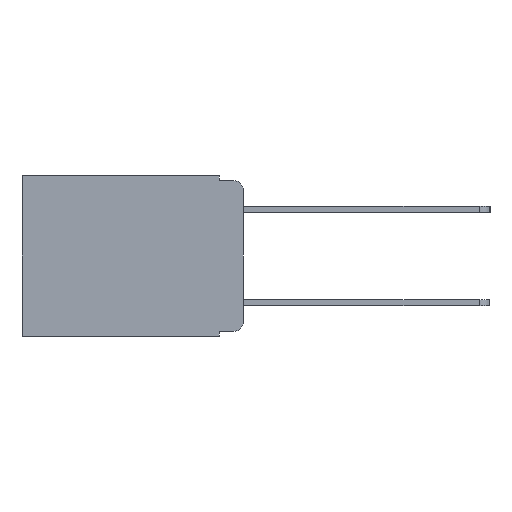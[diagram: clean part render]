
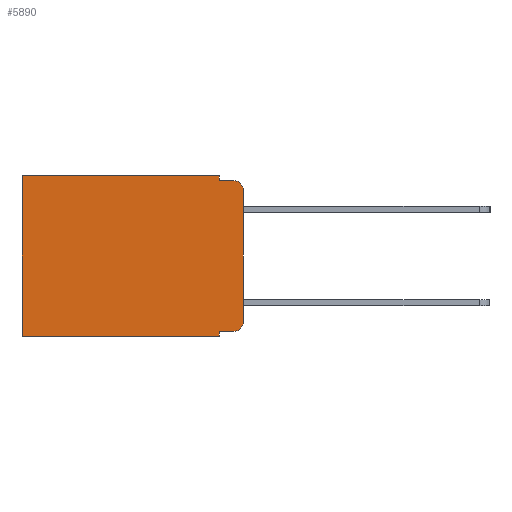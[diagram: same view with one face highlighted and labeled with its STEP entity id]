
A CAD part, left-side view. The second image highlights one B-rep face of the part: STEP entity #5890.
In plain terms, the highlighted planar face has unit normal (-1, 0, 0).
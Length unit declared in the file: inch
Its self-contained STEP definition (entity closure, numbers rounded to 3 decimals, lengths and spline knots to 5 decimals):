
#100 = CARTESIAN_POINT ( 'NONE',  ( 0.298, 0., 0. ) ) ;
#235 = VERTEX_POINT ( 'NONE', #10505 ) ;
#363 = ORIENTED_EDGE ( 'NONE', *, *, #10408, .T. ) ;
#366 = EDGE_CURVE ( 'NONE', #2660, #1047, #8768, .T. ) ;
#435 = EDGE_CURVE ( 'NONE', #1934, #4806, #10610, .T. ) ;
#436 = ORIENTED_EDGE ( 'NONE', *, *, #435, .T. ) ;
#589 = VECTOR ( 'NONE', #9403, 39.37008 ) ;
#624 = ORIENTED_EDGE ( 'NONE', *, *, #366, .F. ) ;
#660 = VERTEX_POINT ( 'NONE', #872 ) ;
#872 = CARTESIAN_POINT ( 'NONE',  ( 0.298, 0.051, -0.333 ) ) ;
#1047 = VERTEX_POINT ( 'NONE', #6591 ) ;
#1181 = DIRECTION ( 'NONE',  ( 0., 0., -1. ) ) ;
#1184 = CARTESIAN_POINT ( 'NONE',  ( 0.298, 0.051, 0. ) ) ;
#1811 = DIRECTION ( 'NONE',  ( 0., 1., 0. ) ) ;
#1934 = VERTEX_POINT ( 'NONE', #4627 ) ;
#2056 = VECTOR ( 'NONE', #4995, 39.37008 ) ;
#2133 = AXIS2_PLACEMENT_3D ( 'NONE', #8592, #3568, #9383 ) ;
#2230 = DIRECTION ( 'NONE',  ( 0., 0., -1. ) ) ;
#2364 = VERTEX_POINT ( 'NONE', #4987 ) ;
#2460 = AXIS2_PLACEMENT_3D ( 'NONE', #4504, #6035, #4057 ) ;
#2660 = VERTEX_POINT ( 'NONE', #5767 ) ;
#2763 = LINE ( 'NONE', #4323, #9146 ) ;
#2935 = LINE ( 'NONE', #100, #589 ) ;
#3089 = AXIS2_PLACEMENT_3D ( 'NONE', #3874, #6316, #7940 ) ;
#3096 = CARTESIAN_POINT ( 'NONE',  ( 0.298, 0.051, 0. ) ) ;
#3352 = CIRCLE ( 'NONE', #2133, 0.02 ) ;
#3515 = ORIENTED_EDGE ( 'NONE', *, *, #6199, .F. ) ;
#3568 = DIRECTION ( 'NONE',  ( -1., 0., 0. ) ) ;
#3852 = LINE ( 'NONE', #9839, #8577 ) ;
#3874 = CARTESIAN_POINT ( 'NONE',  ( 0.298, 0.02, -0.313 ) ) ;
#4001 = LINE ( 'NONE', #10686, #8207 ) ;
#4057 = DIRECTION ( 'NONE',  ( 0., 0., -1. ) ) ;
#4323 = CARTESIAN_POINT ( 'NONE',  ( 0.298, 0., 0. ) ) ;
#4504 = CARTESIAN_POINT ( 'NONE',  ( 0.298, 0., 0. ) ) ;
#4610 = CARTESIAN_POINT ( 'NONE',  ( 0.298, 0., -0.03 ) ) ;
#4627 = CARTESIAN_POINT ( 'NONE',  ( 0.298, 0.02, -0.333 ) ) ;
#4632 = VECTOR ( 'NONE', #2230, 39.37008 ) ;
#4806 = VERTEX_POINT ( 'NONE', #10694 ) ;
#4987 = CARTESIAN_POINT ( 'NONE',  ( 0.298, 0.051, 0. ) ) ;
#4995 = DIRECTION ( 'NONE',  ( 0., 1., 0. ) ) ;
#5471 = LINE ( 'NONE', #1184, #6018 ) ;
#5699 = VERTEX_POINT ( 'NONE', #10056 ) ;
#5726 = DIRECTION ( 'NONE',  ( 0., -1., 0. ) ) ;
#5732 = CARTESIAN_POINT ( 'NONE',  ( 0.298, 0., -0.343 ) ) ;
#5767 = CARTESIAN_POINT ( 'NONE',  ( 0.298, 0.051, -0.343 ) ) ;
#5837 = DIRECTION ( 'NONE',  ( 0., 0., -1. ) ) ;
#5890 = ADVANCED_FACE ( 'NONE', ( #9363 ), #7593, .F. ) ;
#5957 = EDGE_CURVE ( 'NONE', #9773, #235, #10722, .T. ) ;
#6018 = VECTOR ( 'NONE', #1181, 39.37008 ) ;
#6035 = DIRECTION ( 'NONE',  ( 1., 0., 0. ) ) ;
#6199 = EDGE_CURVE ( 'NONE', #2364, #9773, #5471, .T. ) ;
#6316 = DIRECTION ( 'NONE',  ( -1., 0., 0. ) ) ;
#6423 = ORIENTED_EDGE ( 'NONE', *, *, #5957, .F. ) ;
#6591 = CARTESIAN_POINT ( 'NONE',  ( 0.298, 0.473, -0.343 ) ) ;
#6660 = ORIENTED_EDGE ( 'NONE', *, *, #8066, .T. ) ;
#6733 = EDGE_LOOP ( 'NONE', ( #8802, #6660, #6423, #3515, #7667, #363, #624, #8379, #7377, #436 ) ) ;
#7128 = VERTEX_POINT ( 'NONE', #4610 ) ;
#7339 = DIRECTION ( 'NONE',  ( 0., -1., 0. ) ) ;
#7377 = ORIENTED_EDGE ( 'NONE', *, *, #8397, .T. ) ;
#7593 = PLANE ( 'NONE',  #2460 ) ;
#7667 = ORIENTED_EDGE ( 'NONE', *, *, #9535, .T. ) ;
#7940 = DIRECTION ( 'NONE',  ( 0., 0., -1. ) ) ;
#8066 = EDGE_CURVE ( 'NONE', #7128, #235, #3352, .T. ) ;
#8132 = CARTESIAN_POINT ( 'NONE',  ( 0.298, 0.051, -0.01 ) ) ;
#8207 = VECTOR ( 'NONE', #5837, 39.37008 ) ;
#8331 = EDGE_CURVE ( 'NONE', #660, #2660, #9065, .T. ) ;
#8379 = ORIENTED_EDGE ( 'NONE', *, *, #8331, .F. ) ;
#8397 = EDGE_CURVE ( 'NONE', #660, #1934, #3852, .T. ) ;
#8577 = VECTOR ( 'NONE', #5726, 39.37008 ) ;
#8592 = CARTESIAN_POINT ( 'NONE',  ( 0.298, 0.02, -0.03 ) ) ;
#8626 = VECTOR ( 'NONE', #7339, 39.37008 ) ;
#8678 = EDGE_CURVE ( 'NONE', #7128, #4806, #2935, .T. ) ;
#8768 = LINE ( 'NONE', #5732, #2056 ) ;
#8802 = ORIENTED_EDGE ( 'NONE', *, *, #8678, .F. ) ;
#9065 = LINE ( 'NONE', #3096, #4632 ) ;
#9146 = VECTOR ( 'NONE', #1811, 39.37008 ) ;
#9363 = FACE_OUTER_BOUND ( 'NONE', #6733, .T. ) ;
#9383 = DIRECTION ( 'NONE',  ( 0., 0., -1. ) ) ;
#9403 = DIRECTION ( 'NONE',  ( 0., 0., -1. ) ) ;
#9496 = CARTESIAN_POINT ( 'NONE',  ( 0.298, 0.051, -0.01 ) ) ;
#9535 = EDGE_CURVE ( 'NONE', #2364, #5699, #2763, .T. ) ;
#9773 = VERTEX_POINT ( 'NONE', #8132 ) ;
#9839 = CARTESIAN_POINT ( 'NONE',  ( 0.298, 0.051, -0.333 ) ) ;
#10056 = CARTESIAN_POINT ( 'NONE',  ( 0.298, 0.473, 0. ) ) ;
#10408 = EDGE_CURVE ( 'NONE', #5699, #1047, #4001, .T. ) ;
#10505 = CARTESIAN_POINT ( 'NONE',  ( 0.298, 0.02, -0.01 ) ) ;
#10610 = CIRCLE ( 'NONE', #3089, 0.02 ) ;
#10686 = CARTESIAN_POINT ( 'NONE',  ( 0.298, 0.473, 0. ) ) ;
#10694 = CARTESIAN_POINT ( 'NONE',  ( 0.298, 0., -0.313 ) ) ;
#10722 = LINE ( 'NONE', #9496, #8626 ) ;
